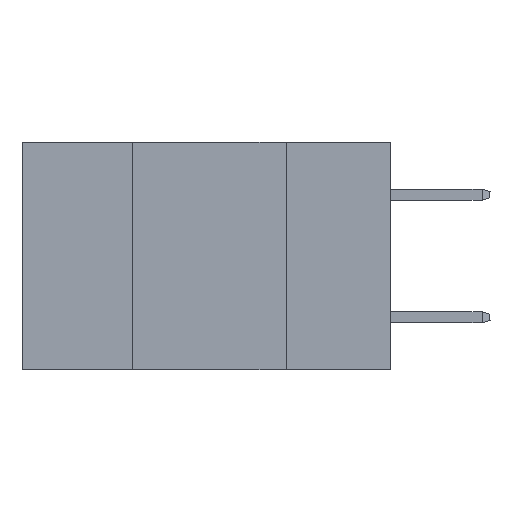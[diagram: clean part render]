
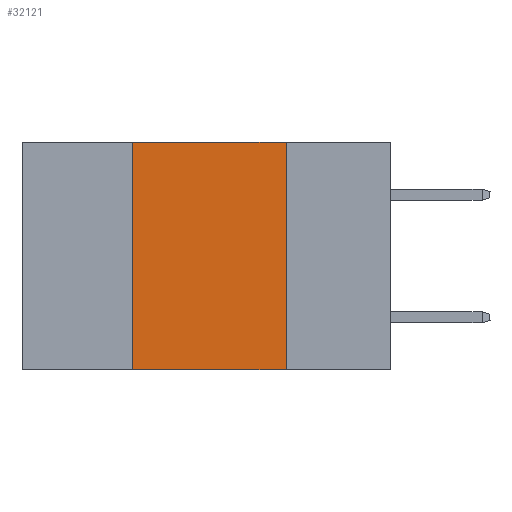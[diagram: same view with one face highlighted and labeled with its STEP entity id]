
A CAD part, left-side view. The second image highlights one B-rep face of the part: STEP entity #32121.
In plain terms, the highlighted planar face has unit normal (-1, 0, 0).
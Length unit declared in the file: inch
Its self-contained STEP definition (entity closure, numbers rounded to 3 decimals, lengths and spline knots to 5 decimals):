
#419 = CARTESIAN_POINT ( 'NONE',  ( 0., 0.6, 0. ) ) ;
#1017 = EDGE_CURVE ( 'NONE', #32006, #20841, #24216, .T. ) ;
#2786 = EDGE_CURVE ( 'NONE', #6085, #22721, #2857, .T. ) ;
#2857 = LINE ( 'NONE', #9883, #13524 ) ;
#3903 = CARTESIAN_POINT ( 'NONE',  ( 0., 0.17, 0. ) ) ;
#4382 = VECTOR ( 'NONE', #27697, 39.37008 ) ;
#5632 = ORIENTED_EDGE ( 'NONE', *, *, #16243, .F. ) ;
#6085 = VERTEX_POINT ( 'NONE', #26091 ) ;
#6558 = ORIENTED_EDGE ( 'NONE', *, *, #2786, .F. ) ;
#6865 = CARTESIAN_POINT ( 'NONE',  ( 0., 0.42, 0. ) ) ;
#7741 = ORIENTED_EDGE ( 'NONE', *, *, #29039, .F. ) ;
#7973 = ORIENTED_EDGE ( 'NONE', *, *, #1017, .T. ) ;
#8934 = DIRECTION ( 'NONE',  ( 0., 0., -1. ) ) ;
#9702 = FACE_OUTER_BOUND ( 'NONE', #22527, .T. ) ;
#9883 = CARTESIAN_POINT ( 'NONE',  ( 0., 0.6, 0. ) ) ;
#10798 = AXIS2_PLACEMENT_3D ( 'NONE', #419, #29220, #13679 ) ;
#11364 = LINE ( 'NONE', #6865, #4382 ) ;
#12630 = DIRECTION ( 'NONE',  ( 0., -1., 0. ) ) ;
#13524 = VECTOR ( 'NONE', #12630, 39.37008 ) ;
#13679 = DIRECTION ( 'NONE',  ( 0., 0., -1. ) ) ;
#15759 = CARTESIAN_POINT ( 'NONE',  ( 0., 0.42, -0.37 ) ) ;
#16243 = EDGE_CURVE ( 'NONE', #22721, #20841, #29583, .T. ) ;
#16503 = VECTOR ( 'NONE', #24399, 39.37008 ) ;
#20841 = VERTEX_POINT ( 'NONE', #26991 ) ;
#21106 = VECTOR ( 'NONE', #8934, 39.37008 ) ;
#21915 = CARTESIAN_POINT ( 'NONE',  ( 0., 0.17, 0. ) ) ;
#22527 = EDGE_LOOP ( 'NONE', ( #5632, #6558, #7741, #7973 ) ) ;
#22721 = VERTEX_POINT ( 'NONE', #3903 ) ;
#24027 = PLANE ( 'NONE',  #10798 ) ;
#24216 = LINE ( 'NONE', #33127, #16503 ) ;
#24399 = DIRECTION ( 'NONE',  ( 0., -1., 0. ) ) ;
#26091 = CARTESIAN_POINT ( 'NONE',  ( 0., 0.42, 0. ) ) ;
#26991 = CARTESIAN_POINT ( 'NONE',  ( 0., 0.17, -0.37 ) ) ;
#27697 = DIRECTION ( 'NONE',  ( 0., 0., 1. ) ) ;
#29039 = EDGE_CURVE ( 'NONE', #32006, #6085, #11364, .T. ) ;
#29220 = DIRECTION ( 'NONE',  ( 1., 0., 0. ) ) ;
#29583 = LINE ( 'NONE', #21915, #21106 ) ;
#32006 = VERTEX_POINT ( 'NONE', #15759 ) ;
#32121 = ADVANCED_FACE ( 'NONE', ( #9702 ), #24027, .F. ) ;
#33127 = CARTESIAN_POINT ( 'NONE',  ( 0., 0.6, -0.37 ) ) ;
